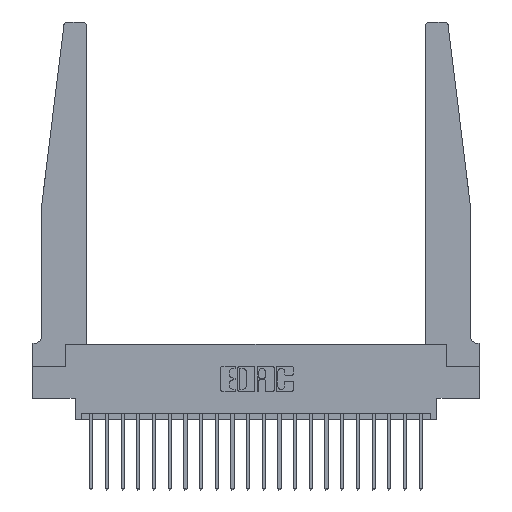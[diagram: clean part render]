
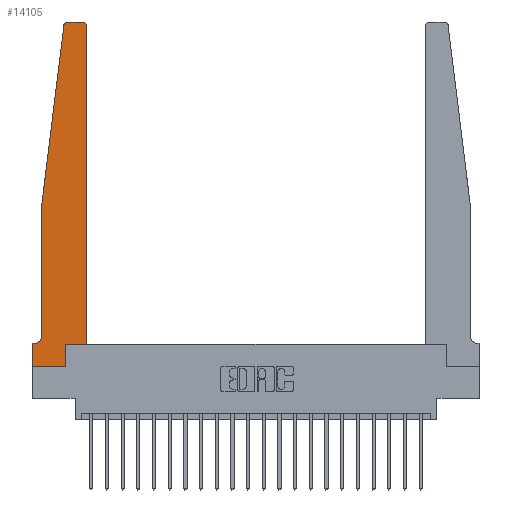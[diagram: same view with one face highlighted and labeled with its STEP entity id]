
A CAD part, top view. The second image highlights one B-rep face of the part: STEP entity #14105.
In plain terms, the highlighted planar face has unit normal (0, 0, 1).
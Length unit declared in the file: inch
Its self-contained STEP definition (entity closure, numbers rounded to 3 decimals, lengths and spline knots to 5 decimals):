
#203 = CARTESIAN_POINT ( 'NONE',  ( 0.425, 0.18, 0.37 ) ) ;
#225 = LINE ( 'NONE', #7265, #11799 ) ;
#582 = CARTESIAN_POINT ( 'NONE',  ( 0.065, 0.1875, 0.37 ) ) ;
#625 = DIRECTION ( 'NONE',  ( 0., -1., 0. ) ) ;
#745 = LINE ( 'NONE', #11061, #11684 ) ;
#819 = CIRCLE ( 'NONE', #8429, 0.03 ) ;
#1278 = CARTESIAN_POINT ( 'NONE',  ( 0., 0., 0.37 ) ) ;
#1606 = LINE ( 'NONE', #15454, #18441 ) ;
#1713 = VERTEX_POINT ( 'NONE', #7986 ) ;
#2188 = VERTEX_POINT ( 'NONE', #18511 ) ;
#2378 = VECTOR ( 'NONE', #4164, 39.37008 ) ;
#2992 = FACE_OUTER_BOUND ( 'NONE', #14513, .T. ) ;
#3727 = DIRECTION ( 'NONE',  ( 1., 0., 0. ) ) ;
#4100 = VERTEX_POINT ( 'NONE', #17904 ) ;
#4164 = DIRECTION ( 'NONE',  ( 0., 1., 0. ) ) ;
#4573 = ORIENTED_EDGE ( 'NONE', *, *, #10963, .T. ) ;
#4687 = ORIENTED_EDGE ( 'NONE', *, *, #15113, .T. ) ;
#4751 = EDGE_CURVE ( 'NONE', #15494, #21179, #19050, .T. ) ;
#4765 = CARTESIAN_POINT ( 'NONE',  ( 0.395, 2.75, 0.37 ) ) ;
#4804 = CARTESIAN_POINT ( 'NONE',  ( 0., 0.1875, 0.37 ) ) ;
#5000 = ORIENTED_EDGE ( 'NONE', *, *, #19652, .T. ) ;
#5083 = ORIENTED_EDGE ( 'NONE', *, *, #4751, .T. ) ;
#5220 = CARTESIAN_POINT ( 'NONE',  ( 0.2605, 0., 0.37 ) ) ;
#5364 = EDGE_CURVE ( 'NONE', #19195, #6774, #16826, .T. ) ;
#5540 = CARTESIAN_POINT ( 'NONE',  ( 0.425, 0.18, 0.37 ) ) ;
#5691 = ORIENTED_EDGE ( 'NONE', *, *, #9823, .T. ) ;
#6389 = AXIS2_PLACEMENT_3D ( 'NONE', #20021, #7541, #19679 ) ;
#6774 = VERTEX_POINT ( 'NONE', #7209 ) ;
#6992 = VERTEX_POINT ( 'NONE', #13323 ) ;
#7086 = EDGE_CURVE ( 'NONE', #14256, #8688, #225, .T. ) ;
#7150 = DIRECTION ( 'NONE',  ( -0.122, -0.992, 0. ) ) ;
#7209 = CARTESIAN_POINT ( 'NONE',  ( 0., 0., 0.37 ) ) ;
#7265 = CARTESIAN_POINT ( 'NONE',  ( 0.065, 1.25, 0.37 ) ) ;
#7541 = DIRECTION ( 'NONE',  ( 0., 0., 1. ) ) ;
#7666 = ORIENTED_EDGE ( 'NONE', *, *, #7086, .T. ) ;
#7682 = ORIENTED_EDGE ( 'NONE', *, *, #11307, .T. ) ;
#7973 = CARTESIAN_POINT ( 'NONE',  ( 0.065, 1.25, 0.37 ) ) ;
#7986 = CARTESIAN_POINT ( 'NONE',  ( 0.425, 0.18, 0.37 ) ) ;
#8075 = ORIENTED_EDGE ( 'NONE', *, *, #9307, .T. ) ;
#8188 = DIRECTION ( 'NONE',  ( 0., -1., 0. ) ) ;
#8429 = AXIS2_PLACEMENT_3D ( 'NONE', #16267, #14229, #14559 ) ;
#8688 = VERTEX_POINT ( 'NONE', #7973 ) ;
#9062 = LINE ( 'NONE', #203, #2378 ) ;
#9280 = VECTOR ( 'NONE', #12720, 39.37008 ) ;
#9307 = EDGE_CURVE ( 'NONE', #8688, #12654, #745, .T. ) ;
#9823 = EDGE_CURVE ( 'NONE', #2188, #14256, #819, .T. ) ;
#10963 = EDGE_CURVE ( 'NONE', #21179, #2188, #14910, .T. ) ;
#11061 = CARTESIAN_POINT ( 'NONE',  ( 0.065, 1.25, 0.37 ) ) ;
#11307 = EDGE_CURVE ( 'NONE', #6774, #12935, #16475, .T. ) ;
#11684 = VECTOR ( 'NONE', #625, 39.37008 ) ;
#11720 = DIRECTION ( 'NONE',  ( 0., 0., 1. ) ) ;
#11799 = VECTOR ( 'NONE', #7150, 39.37008 ) ;
#12654 = VERTEX_POINT ( 'NONE', #14764 ) ;
#12720 = DIRECTION ( 'NONE',  ( -1., 0., 0. ) ) ;
#12833 = DIRECTION ( 'NONE',  ( 1., 0., 0. ) ) ;
#12935 = VERTEX_POINT ( 'NONE', #5220 ) ;
#12947 = CARTESIAN_POINT ( 'NONE',  ( 0.24675, 2.72367, 0.37 ) ) ;
#13069 = LINE ( 'NONE', #582, #9280 ) ;
#13100 = DIRECTION ( 'NONE',  ( -1., 0., 0. ) ) ;
#13200 = DIRECTION ( 'NONE',  ( -1., 0., 0. ) ) ;
#13323 = CARTESIAN_POINT ( 'NONE',  ( 0.2605, 0.18, 0.37 ) ) ;
#13427 = PLANE ( 'NONE',  #19726 ) ;
#13591 = CARTESIAN_POINT ( 'NONE',  ( 0.425, 2.72, 0.37 ) ) ;
#13756 = ORIENTED_EDGE ( 'NONE', *, *, #5364, .T. ) ;
#13942 = CIRCLE ( 'NONE', #20449, 0.05 ) ;
#14076 = EDGE_CURVE ( 'NONE', #12654, #4100, #13942, .T. ) ;
#14105 = ADVANCED_FACE ( 'NONE', ( #2992 ), #13427, .T. ) ;
#14229 = DIRECTION ( 'NONE',  ( 0., 0., 1. ) ) ;
#14256 = VERTEX_POINT ( 'NONE', #12947 ) ;
#14513 = EDGE_LOOP ( 'NONE', ( #4573, #5691, #7666, #8075, #17843, #20681, #13756, #7682, #5000, #16739, #4687, #5083 ) ) ;
#14559 = DIRECTION ( 'NONE',  ( 1., 0., 0. ) ) ;
#14764 = CARTESIAN_POINT ( 'NONE',  ( 0.065, 0.2375, 0.37 ) ) ;
#14910 = LINE ( 'NONE', #19769, #17542 ) ;
#15113 = EDGE_CURVE ( 'NONE', #1713, #15494, #9062, .T. ) ;
#15454 = CARTESIAN_POINT ( 'NONE',  ( 0.2605, 0.18, 0.37 ) ) ;
#15494 = VERTEX_POINT ( 'NONE', #13591 ) ;
#15599 = CARTESIAN_POINT ( 'NONE',  ( 0., 0.1875, 0.37 ) ) ;
#16098 = DIRECTION ( 'NONE',  ( 0., 1., 0. ) ) ;
#16267 = CARTESIAN_POINT ( 'NONE',  ( 0.27653, 2.72, 0.37 ) ) ;
#16403 = EDGE_CURVE ( 'NONE', #4100, #19195, #13069, .T. ) ;
#16475 = LINE ( 'NONE', #21563, #18970 ) ;
#16738 = CARTESIAN_POINT ( 'NONE',  ( 0.015, 0.2375, 0.37 ) ) ;
#16739 = ORIENTED_EDGE ( 'NONE', *, *, #18484, .T. ) ;
#16826 = LINE ( 'NONE', #1278, #19474 ) ;
#17326 = VECTOR ( 'NONE', #3727, 39.37008 ) ;
#17542 = VECTOR ( 'NONE', #13200, 39.37008 ) ;
#17843 = ORIENTED_EDGE ( 'NONE', *, *, #14076, .T. ) ;
#17904 = CARTESIAN_POINT ( 'NONE',  ( 0.015, 0.1875, 0.37 ) ) ;
#18441 = VECTOR ( 'NONE', #16098, 39.37008 ) ;
#18484 = EDGE_CURVE ( 'NONE', #6992, #1713, #20752, .T. ) ;
#18511 = CARTESIAN_POINT ( 'NONE',  ( 0.27653, 2.75, 0.37 ) ) ;
#18645 = DIRECTION ( 'NONE',  ( 1., 0., 0. ) ) ;
#18970 = VECTOR ( 'NONE', #12833, 39.37008 ) ;
#19050 = CIRCLE ( 'NONE', #6389, 0.03 ) ;
#19195 = VERTEX_POINT ( 'NONE', #15599 ) ;
#19474 = VECTOR ( 'NONE', #8188, 39.37008 ) ;
#19652 = EDGE_CURVE ( 'NONE', #12935, #6992, #1606, .T. ) ;
#19679 = DIRECTION ( 'NONE',  ( 1., 0., 0. ) ) ;
#19726 = AXIS2_PLACEMENT_3D ( 'NONE', #4804, #11720, #18645 ) ;
#19769 = CARTESIAN_POINT ( 'NONE',  ( 0.25, 2.75, 0.37 ) ) ;
#20021 = CARTESIAN_POINT ( 'NONE',  ( 0.395, 2.72, 0.37 ) ) ;
#20232 = DIRECTION ( 'NONE',  ( 0., 0., -1. ) ) ;
#20449 = AXIS2_PLACEMENT_3D ( 'NONE', #16738, #20232, #13100 ) ;
#20681 = ORIENTED_EDGE ( 'NONE', *, *, #16403, .T. ) ;
#20752 = LINE ( 'NONE', #5540, #17326 ) ;
#21179 = VERTEX_POINT ( 'NONE', #4765 ) ;
#21563 = CARTESIAN_POINT ( 'NONE',  ( 0., 0., 0.37 ) ) ;
